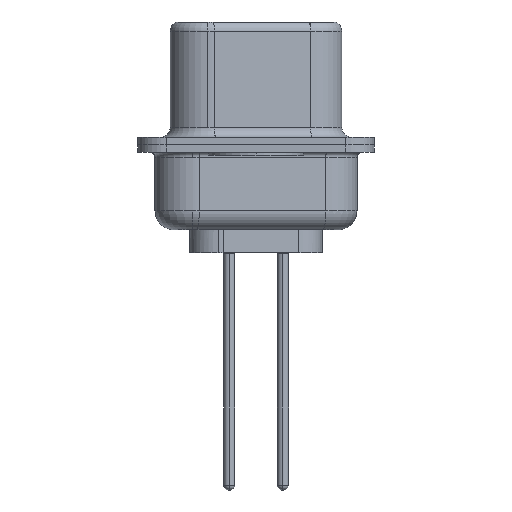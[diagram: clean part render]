
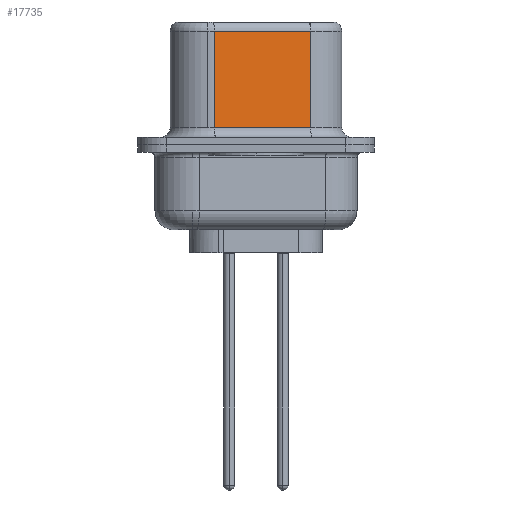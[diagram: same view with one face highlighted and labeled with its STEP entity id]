
A CAD part, left-side view. The second image highlights one B-rep face of the part: STEP entity #17735.
In plain terms, the highlighted planar face has unit normal (-0.985, -0.174, 0).
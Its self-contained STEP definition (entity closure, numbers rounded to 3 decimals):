
#551 = EDGE_CURVE ( 'NONE', #21147, #23004, #11609, .T. ) ;
#827 = ORIENTED_EDGE ( 'NONE', *, *, #1840, .T. ) ;
#1218 = PLANE ( 'NONE',  #18589 ) ;
#1227 = EDGE_CURVE ( 'NONE', #2771, #23004, #22352, .T. ) ;
#1840 = EDGE_CURVE ( 'NONE', #21147, #16119, #7282, .T. ) ;
#2771 = VERTEX_POINT ( 'NONE', #5922 ) ;
#2996 = FACE_OUTER_BOUND ( 'NONE', #7367, .T. ) ;
#3117 = DIRECTION ( 'NONE',  ( -0.174, 0.985, 0. ) ) ;
#3654 = VECTOR ( 'NONE', #4645, 1000. ) ;
#3713 = DIRECTION ( 'NONE',  ( 0., 0., -1. ) ) ;
#3989 = DIRECTION ( 'NONE',  ( -0.174, 0.985, 0. ) ) ;
#4217 = DIRECTION ( 'NONE',  ( 0., 0., -1. ) ) ;
#4645 = DIRECTION ( 'NONE',  ( 0.174, -0.985, 0. ) ) ;
#5639 = CARTESIAN_POINT ( 'NONE',  ( 4.58, -2.897, 6.02 ) ) ;
#5922 = CARTESIAN_POINT ( 'NONE',  ( 3.68, 2.203, 0.9 ) ) ;
#7282 = LINE ( 'NONE', #5639, #12373 ) ;
#7367 = EDGE_LOOP ( 'NONE', ( #21090, #827, #9917, #11643 ) ) ;
#8392 = CARTESIAN_POINT ( 'NONE',  ( 4.58, -2.897, 6.52 ) ) ;
#8512 = DIRECTION ( 'NONE',  ( 0.985, 0.174, 0. ) ) ;
#8536 = CARTESIAN_POINT ( 'NONE',  ( 4.58, -2.897, 0.9 ) ) ;
#9321 = EDGE_CURVE ( 'NONE', #16119, #2771, #10536, .T. ) ;
#9917 = ORIENTED_EDGE ( 'NONE', *, *, #9321, .T. ) ;
#10536 = LINE ( 'NONE', #19417, #21047 ) ;
#11431 = CARTESIAN_POINT ( 'NONE',  ( 4.58, -2.897, 6.02 ) ) ;
#11609 = LINE ( 'NONE', #13146, #22545 ) ;
#11643 = ORIENTED_EDGE ( 'NONE', *, *, #1227, .T. ) ;
#12373 = VECTOR ( 'NONE', #3989, 1000. ) ;
#13146 = CARTESIAN_POINT ( 'NONE',  ( 4.58, -2.897, 6.52 ) ) ;
#16119 = VERTEX_POINT ( 'NONE', #16201 ) ;
#16201 = CARTESIAN_POINT ( 'NONE',  ( 3.68, 2.203, 6.02 ) ) ;
#17411 = CARTESIAN_POINT ( 'NONE',  ( 4.58, -2.897, 0.9 ) ) ;
#17735 = ADVANCED_FACE ( 'NONE', ( #2996 ), #1218, .F. ) ;
#18589 = AXIS2_PLACEMENT_3D ( 'NONE', #8392, #8512, #3117 ) ;
#19417 = CARTESIAN_POINT ( 'NONE',  ( 3.68, 2.203, 6.52 ) ) ;
#21047 = VECTOR ( 'NONE', #3713, 1000. ) ;
#21090 = ORIENTED_EDGE ( 'NONE', *, *, #551, .F. ) ;
#21147 = VERTEX_POINT ( 'NONE', #11431 ) ;
#22352 = LINE ( 'NONE', #17411, #3654 ) ;
#22545 = VECTOR ( 'NONE', #4217, 1000. ) ;
#23004 = VERTEX_POINT ( 'NONE', #8536 ) ;
